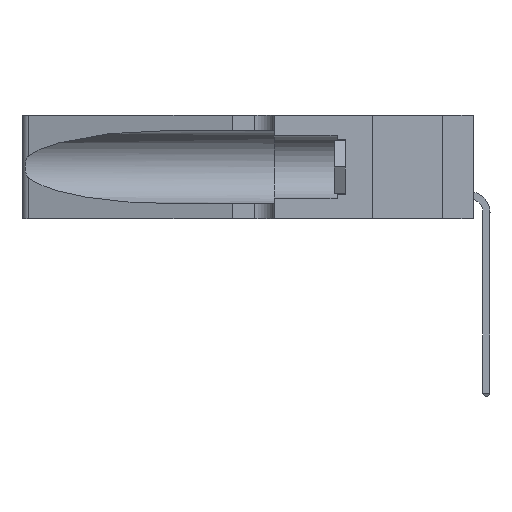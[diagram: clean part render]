
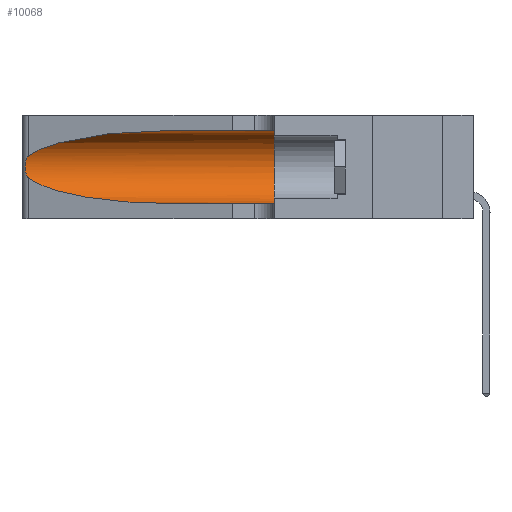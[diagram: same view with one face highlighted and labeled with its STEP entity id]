
A CAD part, left-side view. The second image highlights one B-rep face of the part: STEP entity #10068.
In plain terms, the highlighted cylindrical face has radius 3.308 mm (diameter 6.617 mm), a partial arc.
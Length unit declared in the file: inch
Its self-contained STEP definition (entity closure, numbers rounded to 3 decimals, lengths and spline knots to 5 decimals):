
#569 = EDGE_CURVE ( 'NONE', #14056, #3779, #5079, .T. ) ;
#696 = VERTEX_POINT ( 'NONE', #27454 ) ;
#1024 = CARTESIAN_POINT ( 'NONE',  ( 0.25639, 1.23186, 0.15144 ) ) ;
#2071 = ORIENTED_EDGE ( 'NONE', *, *, #15743, .T. ) ;
#2248 =( BOUNDED_CURVE ( )  B_SPLINE_CURVE ( 3, ( #24410, #6929, #12236, #19813 ),
 .UNSPECIFIED., .F., .F. ) 
 B_SPLINE_CURVE_WITH_KNOTS ( ( 4, 4 ),
 ( 3.44316, 4.71239 ),
 .UNSPECIFIED. ) 
 CURVE ( )  GEOMETRIC_REPRESENTATION_ITEM ( )  RATIONAL_B_SPLINE_CURVE ( ( 1., 0.87, 0.87, 1. ) ) 
 REPRESENTATION_ITEM ( '' )  );
#3536 = ORIENTED_EDGE ( 'NONE', *, *, #569, .F. ) ;
#3731 = CARTESIAN_POINT ( 'NONE',  ( 0.25639, 1.23184, 0.21858 ) ) ;
#3779 = VERTEX_POINT ( 'NONE', #19906 ) ;
#3846 = CARTESIAN_POINT ( 'NONE',  ( 0.26075, 1.23896, 0.19203 ) ) ;
#4091 = DIRECTION ( 'NONE',  ( 0., -1., 0. ) ) ;
#5079 = LINE ( 'NONE', #21913, #11512 ) ;
#5320 = VECTOR ( 'NONE', #4091, 39.37008 ) ;
#5353 = CARTESIAN_POINT ( 'NONE',  ( 0.1305, 0.72297, 0.31525 ) ) ;
#5461 = CARTESIAN_POINT ( 'NONE',  ( 0.2373, 1.15595, 0.28018 ) ) ;
#5510 = EDGE_CURVE ( 'NONE', #15523, #696, #9684, .T. ) ;
#6929 = CARTESIAN_POINT ( 'NONE',  ( 0.2373, 1.15595, 0.08982 ) ) ;
#8449 = DIRECTION ( 'NONE',  ( 0., 0., 1. ) ) ;
#8906 = CARTESIAN_POINT ( 'NONE',  ( 0.26017, 1.23833, 0.17102 ) ) ;
#9124 = CARTESIAN_POINT ( 'NONE',  ( 0.25789, 1.23486, 0.15765 ) ) ;
#9368 = VERTEX_POINT ( 'NONE', #32362 ) ;
#9684 = B_SPLINE_CURVE_WITH_KNOTS ( 'NONE', 3,
 ( #32103, #14318, #3731, #14091, #21986, #13983, #3846, #24564, #8906, #11719, #9124, #1024, #29743, #11605 ),
 .UNSPECIFIED., .F., .F.,
 ( 4, 2, 2, 2, 2, 2, 4 ),
 ( 0., 0.00027, 0.00053, 0.00107, 0.0016, 0.00187, 0.00214 ),
 .UNSPECIFIED. ) ;
#10068 = ADVANCED_FACE ( 'NONE', ( #12044 ), #15675, .F. ) ;
#10450 = CIRCLE ( 'NONE', #15120, 0.13025 ) ;
#11512 = VECTOR ( 'NONE', #32030, 39.37008 ) ;
#11605 = CARTESIAN_POINT ( 'NONE',  ( 0.25487, 1.22718, 0.14631 ) ) ;
#11719 = CARTESIAN_POINT ( 'NONE',  ( 0.25856, 1.23593, 0.16098 ) ) ;
#12044 = FACE_OUTER_BOUND ( 'NONE', #18642, .T. ) ;
#12236 = CARTESIAN_POINT ( 'NONE',  ( 0.18966, 0.96281, 0.05475 ) ) ;
#13983 = CARTESIAN_POINT ( 'NONE',  ( 0.26018, 1.23835, 0.19895 ) ) ;
#14056 = VERTEX_POINT ( 'NONE', #28268 ) ;
#14091 = CARTESIAN_POINT ( 'NONE',  ( 0.25787, 1.23484, 0.2124 ) ) ;
#14318 = CARTESIAN_POINT ( 'NONE',  ( 0.25555, 1.22994, 0.2215 ) ) ;
#14418 = CARTESIAN_POINT ( 'NONE',  ( 0.1305, 1.61858, 0.185 ) ) ;
#15120 = AXIS2_PLACEMENT_3D ( 'NONE', #31436, #21110, #8449 ) ;
#15523 = VERTEX_POINT ( 'NONE', #18127 ) ;
#15675 = CYLINDRICAL_SURFACE ( 'NONE', #17597, 0.13025 ) ;
#15714 = CARTESIAN_POINT ( 'NONE',  ( 0.18966, 0.96281, 0.31525 ) ) ;
#15743 = EDGE_CURVE ( 'NONE', #696, #25847, #2248, .T. ) ;
#16723 = EDGE_CURVE ( 'NONE', #3779, #9368, #10450, .T. ) ;
#17597 = AXIS2_PLACEMENT_3D ( 'NONE', #14418, #31995, #21773 ) ;
#17711 = ORIENTED_EDGE ( 'NONE', *, *, #5510, .T. ) ;
#18071 = ORIENTED_EDGE ( 'NONE', *, *, #23456, .T. ) ;
#18127 = CARTESIAN_POINT ( 'NONE',  ( 0.25487, 1.22718, 0.22369 ) ) ;
#18642 = EDGE_LOOP ( 'NONE', ( #30034, #17711, #2071, #18071, #31329, #3536 ) ) ;
#19760 = CARTESIAN_POINT ( 'NONE',  ( 0.1305, 1.61858, 0.05475 ) ) ;
#19813 = CARTESIAN_POINT ( 'NONE',  ( 0.1305, 0.72297, 0.05475 ) ) ;
#19906 = CARTESIAN_POINT ( 'NONE',  ( 0.1305, 0.35, 0.31525 ) ) ;
#21027 = CARTESIAN_POINT ( 'NONE',  ( 0.25487, 1.22718, 0.22369 ) ) ;
#21110 = DIRECTION ( 'NONE',  ( 0., 1., 0. ) ) ;
#21773 = DIRECTION ( 'NONE',  ( 0., 0., -1. ) ) ;
#21913 = CARTESIAN_POINT ( 'NONE',  ( 0.1305, 1.61858, 0.31525 ) ) ;
#21986 = CARTESIAN_POINT ( 'NONE',  ( 0.25854, 1.2359, 0.20912 ) ) ;
#23217 = CARTESIAN_POINT ( 'NONE',  ( 0.1305, 0.72297, 0.05475 ) ) ;
#23456 = EDGE_CURVE ( 'NONE', #25847, #9368, #23859, .T. ) ;
#23859 = LINE ( 'NONE', #19760, #5320 ) ;
#24410 = CARTESIAN_POINT ( 'NONE',  ( 0.25487, 1.22718, 0.14631 ) ) ;
#24564 = CARTESIAN_POINT ( 'NONE',  ( 0.26075, 1.23896, 0.178 ) ) ;
#25847 = VERTEX_POINT ( 'NONE', #23217 ) ;
#27454 = CARTESIAN_POINT ( 'NONE',  ( 0.25487, 1.22718, 0.14631 ) ) ;
#27644 =( BOUNDED_CURVE ( )  B_SPLINE_CURVE ( 3, ( #5353, #15714, #5461, #21027 ),
 .UNSPECIFIED., .F., .T. ) 
 B_SPLINE_CURVE_WITH_KNOTS ( ( 4, 4 ),
 ( 1.5708, 2.84003 ),
 .UNSPECIFIED. ) 
 CURVE ( )  GEOMETRIC_REPRESENTATION_ITEM ( )  RATIONAL_B_SPLINE_CURVE ( ( 1., 0.87, 0.87, 1. ) ) 
 REPRESENTATION_ITEM ( '' )  );
#28268 = CARTESIAN_POINT ( 'NONE',  ( 0.1305, 0.72297, 0.31525 ) ) ;
#29743 = CARTESIAN_POINT ( 'NONE',  ( 0.25555, 1.22993, 0.14849 ) ) ;
#30034 = ORIENTED_EDGE ( 'NONE', *, *, #33239, .T. ) ;
#31329 = ORIENTED_EDGE ( 'NONE', *, *, #16723, .F. ) ;
#31436 = CARTESIAN_POINT ( 'NONE',  ( 0.1305, 0.35, 0.185 ) ) ;
#31995 = DIRECTION ( 'NONE',  ( 0., -1., 0. ) ) ;
#32030 = DIRECTION ( 'NONE',  ( 0., -1., 0. ) ) ;
#32103 = CARTESIAN_POINT ( 'NONE',  ( 0.25487, 1.22718, 0.22369 ) ) ;
#32362 = CARTESIAN_POINT ( 'NONE',  ( 0.1305, 0.35, 0.05475 ) ) ;
#33239 = EDGE_CURVE ( 'NONE', #14056, #15523, #27644, .T. ) ;
